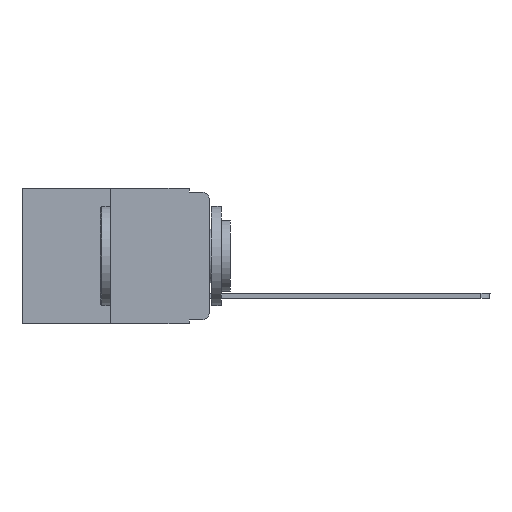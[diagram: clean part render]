
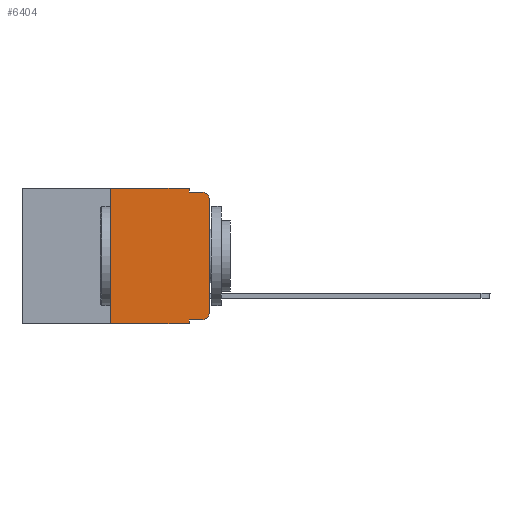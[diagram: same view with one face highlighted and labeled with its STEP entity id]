
A CAD part, left-side view. The second image highlights one B-rep face of the part: STEP entity #6404.
In plain terms, the highlighted planar face has unit normal (-1, 0, 0).
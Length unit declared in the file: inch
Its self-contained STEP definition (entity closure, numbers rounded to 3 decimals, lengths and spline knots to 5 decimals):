
#160 = CARTESIAN_POINT ( 'NONE',  ( 0., 0., -0.313 ) ) ;
#254 = CARTESIAN_POINT ( 'NONE',  ( 0., 0.051, -0.333 ) ) ;
#817 = ORIENTED_EDGE ( 'NONE', *, *, #3560, .T. ) ;
#848 = CIRCLE ( 'NONE', #12452, 0.02 ) ;
#986 = LINE ( 'NONE', #12984, #12958 ) ;
#1222 = DIRECTION ( 'NONE',  ( 0., 0., -1. ) ) ;
#1330 = ORIENTED_EDGE ( 'NONE', *, *, #5449, .T. ) ;
#1384 = DIRECTION ( 'NONE',  ( -1., 0., 0. ) ) ;
#1428 = DIRECTION ( 'NONE',  ( 0., 0., -1. ) ) ;
#1729 = VERTEX_POINT ( 'NONE', #6080 ) ;
#1940 = EDGE_CURVE ( 'NONE', #13736, #6469, #4348, .T. ) ;
#2114 = LINE ( 'NONE', #8129, #6343 ) ;
#2296 = DIRECTION ( 'NONE',  ( 0., 0., -1. ) ) ;
#2310 = VERTEX_POINT ( 'NONE', #13199 ) ;
#2339 = DIRECTION ( 'NONE',  ( 0., 0., -1. ) ) ;
#2809 = CARTESIAN_POINT ( 'NONE',  ( 0., 0., -0.03 ) ) ;
#2874 = CARTESIAN_POINT ( 'NONE',  ( 0., 0.051, -0.343 ) ) ;
#2898 = EDGE_CURVE ( 'NONE', #6993, #1729, #11745, .T. ) ;
#3030 = CARTESIAN_POINT ( 'NONE',  ( 0., 0.051, -0.01 ) ) ;
#3247 = DIRECTION ( 'NONE',  ( 0., 0., 1. ) ) ;
#3560 = EDGE_CURVE ( 'NONE', #6469, #12943, #2114, .T. ) ;
#3638 = EDGE_CURVE ( 'NONE', #12943, #2310, #848, .T. ) ;
#4299 = LINE ( 'NONE', #3030, #8891 ) ;
#4348 = CIRCLE ( 'NONE', #11573, 0.02 ) ;
#4392 = DIRECTION ( 'NONE',  ( 0., 0., 1. ) ) ;
#4681 = DIRECTION ( 'NONE',  ( 1., 0., 0. ) ) ;
#4942 = EDGE_CURVE ( 'NONE', #11961, #6730, #986, .T. ) ;
#5138 = ORIENTED_EDGE ( 'NONE', *, *, #4942, .F. ) ;
#5208 = DIRECTION ( 'NONE',  ( 0., 0., -1. ) ) ;
#5449 = EDGE_CURVE ( 'NONE', #13423, #13736, #10423, .T. ) ;
#5609 = CARTESIAN_POINT ( 'NONE',  ( 0., 0.02, -0.333 ) ) ;
#5662 = CARTESIAN_POINT ( 'NONE',  ( 0., 0.25, 0. ) ) ;
#5946 = DIRECTION ( 'NONE',  ( 0., -1., 0. ) ) ;
#6080 = CARTESIAN_POINT ( 'NONE',  ( 0., 0.25, 0. ) ) ;
#6177 = VECTOR ( 'NONE', #4392, 39.37008 ) ;
#6283 = ORIENTED_EDGE ( 'NONE', *, *, #1940, .T. ) ;
#6343 = VECTOR ( 'NONE', #3247, 39.37008 ) ;
#6404 = ADVANCED_FACE ( 'NONE', ( #9494 ), #13782, .F. ) ;
#6469 = VERTEX_POINT ( 'NONE', #160 ) ;
#6500 = ORIENTED_EDGE ( 'NONE', *, *, #3638, .T. ) ;
#6533 = DIRECTION ( 'NONE',  ( 0., -1., 0. ) ) ;
#6730 = VERTEX_POINT ( 'NONE', #13576 ) ;
#6880 = CARTESIAN_POINT ( 'NONE',  ( 0., 0.473, 0. ) ) ;
#6993 = VERTEX_POINT ( 'NONE', #9659 ) ;
#7817 = LINE ( 'NONE', #9293, #8890 ) ;
#8129 = CARTESIAN_POINT ( 'NONE',  ( 0., 0., 0. ) ) ;
#8659 = ORIENTED_EDGE ( 'NONE', *, *, #2898, .F. ) ;
#8662 = CARTESIAN_POINT ( 'NONE',  ( 0., 0.02, -0.313 ) ) ;
#8890 = VECTOR ( 'NONE', #2296, 39.37008 ) ;
#8891 = VECTOR ( 'NONE', #6533, 39.37008 ) ;
#9185 = EDGE_CURVE ( 'NONE', #13423, #11085, #7817, .T. ) ;
#9293 = CARTESIAN_POINT ( 'NONE',  ( 0., 0.051, 0. ) ) ;
#9494 = FACE_OUTER_BOUND ( 'NONE', #12815, .T. ) ;
#9659 = CARTESIAN_POINT ( 'NONE',  ( 0., 0.25, -0.343 ) ) ;
#9866 = DIRECTION ( 'NONE',  ( 0., -1., 0. ) ) ;
#10423 = LINE ( 'NONE', #254, #12748 ) ;
#10476 = CARTESIAN_POINT ( 'NONE',  ( 0., 0.02, -0.03 ) ) ;
#11085 = VERTEX_POINT ( 'NONE', #2874 ) ;
#11281 = EDGE_CURVE ( 'NONE', #6730, #2310, #4299, .T. ) ;
#11324 = ORIENTED_EDGE ( 'NONE', *, *, #11908, .T. ) ;
#11573 = AXIS2_PLACEMENT_3D ( 'NONE', #8662, #14456, #5208 ) ;
#11745 = LINE ( 'NONE', #5662, #6177 ) ;
#11884 = VECTOR ( 'NONE', #14848, 39.37008 ) ;
#11908 = EDGE_CURVE ( 'NONE', #6993, #11085, #14048, .T. ) ;
#11961 = VERTEX_POINT ( 'NONE', #12566 ) ;
#12356 = EDGE_CURVE ( 'NONE', #1729, #11961, #14756, .T. ) ;
#12452 = AXIS2_PLACEMENT_3D ( 'NONE', #10476, #1384, #1222 ) ;
#12566 = CARTESIAN_POINT ( 'NONE',  ( 0., 0.051, 0. ) ) ;
#12748 = VECTOR ( 'NONE', #5946, 39.37008 ) ;
#12815 = EDGE_LOOP ( 'NONE', ( #817, #6500, #13623, #5138, #14541, #8659, #11324, #13361, #1330, #6283 ) ) ;
#12943 = VERTEX_POINT ( 'NONE', #2809 ) ;
#12958 = VECTOR ( 'NONE', #1428, 39.37008 ) ;
#12984 = CARTESIAN_POINT ( 'NONE',  ( 0., 0.051, 0. ) ) ;
#13199 = CARTESIAN_POINT ( 'NONE',  ( 0., 0.02, -0.01 ) ) ;
#13236 = CARTESIAN_POINT ( 'NONE',  ( 0., 0.473, 0. ) ) ;
#13361 = ORIENTED_EDGE ( 'NONE', *, *, #9185, .F. ) ;
#13423 = VERTEX_POINT ( 'NONE', #14139 ) ;
#13576 = CARTESIAN_POINT ( 'NONE',  ( 0., 0.051, -0.01 ) ) ;
#13623 = ORIENTED_EDGE ( 'NONE', *, *, #11281, .F. ) ;
#13732 = CARTESIAN_POINT ( 'NONE',  ( 0., 0.473, -0.343 ) ) ;
#13736 = VERTEX_POINT ( 'NONE', #5609 ) ;
#13782 = PLANE ( 'NONE',  #14503 ) ;
#13848 = VECTOR ( 'NONE', #9866, 39.37008 ) ;
#14048 = LINE ( 'NONE', #13732, #11884 ) ;
#14139 = CARTESIAN_POINT ( 'NONE',  ( 0., 0.051, -0.333 ) ) ;
#14456 = DIRECTION ( 'NONE',  ( -1., 0., 0. ) ) ;
#14503 = AXIS2_PLACEMENT_3D ( 'NONE', #6880, #4681, #2339 ) ;
#14541 = ORIENTED_EDGE ( 'NONE', *, *, #12356, .F. ) ;
#14756 = LINE ( 'NONE', #13236, #13848 ) ;
#14848 = DIRECTION ( 'NONE',  ( 0., -1., 0. ) ) ;
